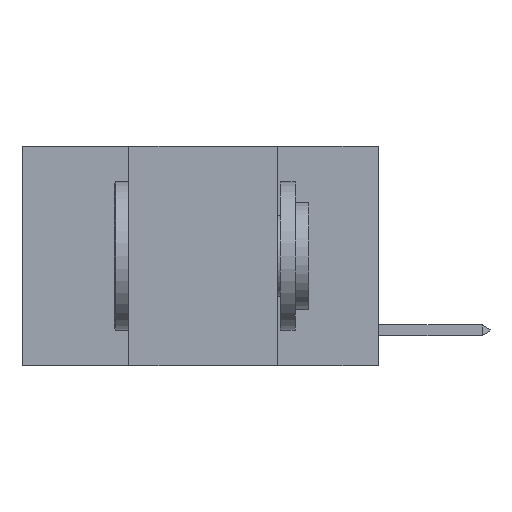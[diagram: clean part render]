
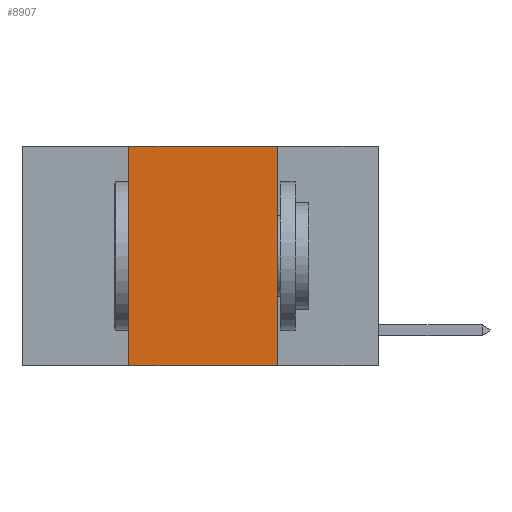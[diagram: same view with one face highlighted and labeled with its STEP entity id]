
A CAD part, left-side view. The second image highlights one B-rep face of the part: STEP entity #8907.
In plain terms, the highlighted planar face has unit normal (-1, 0, 0).
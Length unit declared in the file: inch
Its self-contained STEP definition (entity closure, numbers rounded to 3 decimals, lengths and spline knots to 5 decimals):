
#1366 = AXIS2_PLACEMENT_3D ( 'NONE', #5660, #19160, #9255 ) ;
#2563 = ORIENTED_EDGE ( 'NONE', *, *, #4737, .F. ) ;
#3804 = DIRECTION ( 'NONE',  ( 0., 0., 1. ) ) ;
#3952 = EDGE_CURVE ( 'NONE', #5873, #19457, #19082, .T. ) ;
#4606 = VERTEX_POINT ( 'NONE', #10295 ) ;
#4737 = EDGE_CURVE ( 'NONE', #5873, #4606, #8701, .T. ) ;
#5173 = EDGE_CURVE ( 'NONE', #4606, #21317, #21410, .T. ) ;
#5660 = CARTESIAN_POINT ( 'NONE',  ( 0., 0.6, 0. ) ) ;
#5873 = VERTEX_POINT ( 'NONE', #18472 ) ;
#6242 = CARTESIAN_POINT ( 'NONE',  ( 0., 0.17, -0.37 ) ) ;
#6262 = VECTOR ( 'NONE', #10220, 39.37008 ) ;
#7442 = PLANE ( 'NONE',  #1366 ) ;
#7521 = DIRECTION ( 'NONE',  ( 0., -1., 0. ) ) ;
#7754 = DIRECTION ( 'NONE',  ( 0., -1., 0. ) ) ;
#8701 = LINE ( 'NONE', #14173, #21905 ) ;
#8907 = ADVANCED_FACE ( 'NONE', ( #21068 ), #7442, .F. ) ;
#9255 = DIRECTION ( 'NONE',  ( 0., 0., -1. ) ) ;
#10220 = DIRECTION ( 'NONE',  ( 0., 0., -1. ) ) ;
#10291 = VECTOR ( 'NONE', #7754, 39.37008 ) ;
#10295 = CARTESIAN_POINT ( 'NONE',  ( 0., 0.42, 0. ) ) ;
#10913 = LINE ( 'NONE', #18483, #6262 ) ;
#12415 = ORIENTED_EDGE ( 'NONE', *, *, #5173, .F. ) ;
#12662 = VECTOR ( 'NONE', #7521, 39.37008 ) ;
#12939 = ORIENTED_EDGE ( 'NONE', *, *, #21370, .F. ) ;
#14173 = CARTESIAN_POINT ( 'NONE',  ( 0., 0.42, 0. ) ) ;
#14548 = EDGE_LOOP ( 'NONE', ( #12939, #12415, #2563, #20141 ) ) ;
#17600 = CARTESIAN_POINT ( 'NONE',  ( 0., 0.6, 0. ) ) ;
#18472 = CARTESIAN_POINT ( 'NONE',  ( 0., 0.42, -0.37 ) ) ;
#18483 = CARTESIAN_POINT ( 'NONE',  ( 0., 0.17, 0. ) ) ;
#19082 = LINE ( 'NONE', #19435, #10291 ) ;
#19160 = DIRECTION ( 'NONE',  ( 1., 0., 0. ) ) ;
#19435 = CARTESIAN_POINT ( 'NONE',  ( 0., 0.6, -0.37 ) ) ;
#19457 = VERTEX_POINT ( 'NONE', #6242 ) ;
#19986 = CARTESIAN_POINT ( 'NONE',  ( 0., 0.17, 0. ) ) ;
#20141 = ORIENTED_EDGE ( 'NONE', *, *, #3952, .T. ) ;
#21068 = FACE_OUTER_BOUND ( 'NONE', #14548, .T. ) ;
#21317 = VERTEX_POINT ( 'NONE', #19986 ) ;
#21370 = EDGE_CURVE ( 'NONE', #21317, #19457, #10913, .T. ) ;
#21410 = LINE ( 'NONE', #17600, #12662 ) ;
#21905 = VECTOR ( 'NONE', #3804, 39.37008 ) ;
